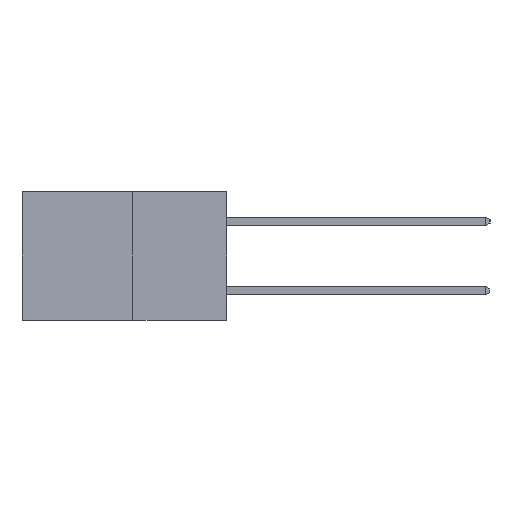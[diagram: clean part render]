
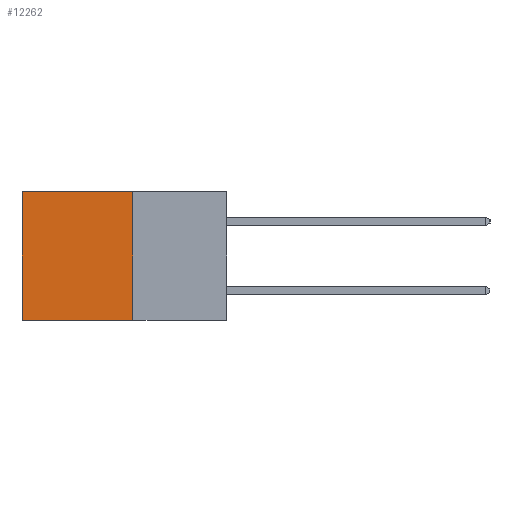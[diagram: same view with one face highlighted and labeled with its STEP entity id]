
A CAD part, left-side view. The second image highlights one B-rep face of the part: STEP entity #12262.
In plain terms, the highlighted planar face has unit normal (-1, 0, 0).
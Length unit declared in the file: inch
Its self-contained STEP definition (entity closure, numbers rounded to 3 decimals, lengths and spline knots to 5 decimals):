
#288 = VECTOR ( 'NONE', #12943, 39.37008 ) ;
#433 = EDGE_CURVE ( 'NONE', #3649, #3344, #8267, .T. ) ;
#1107 = DIRECTION ( 'NONE',  ( 0., 0., -1. ) ) ;
#1181 = CARTESIAN_POINT ( 'NONE',  ( 0.277, 0.27, -0.37 ) ) ;
#1238 = VERTEX_POINT ( 'NONE', #9189 ) ;
#1243 = CARTESIAN_POINT ( 'NONE',  ( 0.277, 0.59, -0.37 ) ) ;
#1439 = CARTESIAN_POINT ( 'NONE',  ( 0.277, 0.27, 0. ) ) ;
#1563 = LINE ( 'NONE', #1181, #4344 ) ;
#1827 = CARTESIAN_POINT ( 'NONE',  ( 0.277, 0.27, -0.37 ) ) ;
#2699 = VECTOR ( 'NONE', #13332, 39.37008 ) ;
#2865 = DIRECTION ( 'NONE',  ( 0., 1., 0. ) ) ;
#3086 = LINE ( 'NONE', #3503, #288 ) ;
#3089 = ORIENTED_EDGE ( 'NONE', *, *, #8880, .T. ) ;
#3344 = VERTEX_POINT ( 'NONE', #1243 ) ;
#3503 = CARTESIAN_POINT ( 'NONE',  ( 0.277, 0.59, -0.37 ) ) ;
#3649 = VERTEX_POINT ( 'NONE', #1827 ) ;
#4344 = VECTOR ( 'NONE', #5329, 39.37008 ) ;
#5092 = VECTOR ( 'NONE', #2865, 39.37008 ) ;
#5227 = ORIENTED_EDGE ( 'NONE', *, *, #433, .F. ) ;
#5329 = DIRECTION ( 'NONE',  ( 0., 0., -1. ) ) ;
#5985 = EDGE_CURVE ( 'NONE', #1238, #3649, #1563, .T. ) ;
#7370 = DIRECTION ( 'NONE',  ( 1., 0., 0. ) ) ;
#7875 = LINE ( 'NONE', #1439, #5092 ) ;
#8267 = LINE ( 'NONE', #9748, #2699 ) ;
#8384 = PLANE ( 'NONE',  #10196 ) ;
#8880 = EDGE_CURVE ( 'NONE', #1238, #9489, #7875, .T. ) ;
#9189 = CARTESIAN_POINT ( 'NONE',  ( 0.277, 0.27, 0. ) ) ;
#9489 = VERTEX_POINT ( 'NONE', #9987 ) ;
#9748 = CARTESIAN_POINT ( 'NONE',  ( 0.277, 0.27, -0.37 ) ) ;
#9987 = CARTESIAN_POINT ( 'NONE',  ( 0.277, 0.59, 0. ) ) ;
#10196 = AXIS2_PLACEMENT_3D ( 'NONE', #10509, #7370, #1107 ) ;
#10509 = CARTESIAN_POINT ( 'NONE',  ( 0.277, 0.27, -0.37 ) ) ;
#11131 = FACE_OUTER_BOUND ( 'NONE', #12059, .T. ) ;
#11140 = ORIENTED_EDGE ( 'NONE', *, *, #5985, .F. ) ;
#11788 = EDGE_CURVE ( 'NONE', #9489, #3344, #3086, .T. ) ;
#12059 = EDGE_LOOP ( 'NONE', ( #12094, #5227, #11140, #3089 ) ) ;
#12094 = ORIENTED_EDGE ( 'NONE', *, *, #11788, .T. ) ;
#12262 = ADVANCED_FACE ( 'NONE', ( #11131 ), #8384, .F. ) ;
#12943 = DIRECTION ( 'NONE',  ( 0., 0., -1. ) ) ;
#13332 = DIRECTION ( 'NONE',  ( 0., 1., 0. ) ) ;
